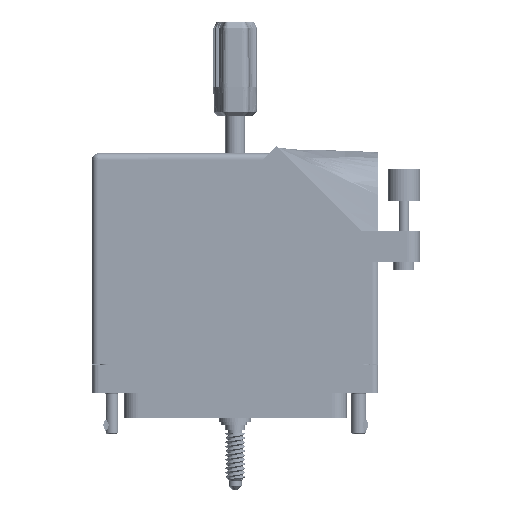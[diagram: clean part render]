
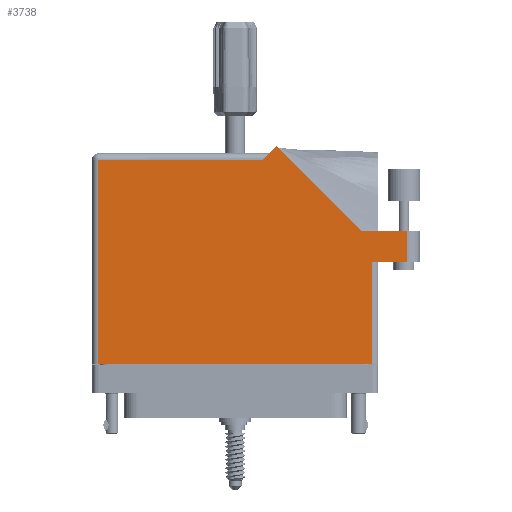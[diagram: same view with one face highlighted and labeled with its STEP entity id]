
A CAD part, front view. The second image highlights one B-rep face of the part: STEP entity #3738.
In plain terms, the highlighted face is planar.
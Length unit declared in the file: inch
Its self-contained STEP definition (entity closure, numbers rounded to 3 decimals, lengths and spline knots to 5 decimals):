
#2102 = ORIENTED_EDGE ( 'NONE', *, *, #64452, .T. ) ;
#3738 = ADVANCED_FACE ( 'NONE', ( #49669 ), #27587, .F. ) ;
#4021 = ORIENTED_EDGE ( 'NONE', *, *, #21366, .T. ) ;
#4444 = EDGE_CURVE ( 'NONE', #12340, #99884, #66323, .T. ) ;
#4753 = ORIENTED_EDGE ( 'NONE', *, *, #93222, .T. ) ;
#4767 = CARTESIAN_POINT ( 'NONE',  ( -1.3155, 1.868, 0.765 ) ) ;
#5941 = DIRECTION ( 'NONE',  ( -1., 0., 0. ) ) ;
#6833 = DIRECTION ( 'NONE',  ( -1., 0., 0. ) ) ;
#11622 = VECTOR ( 'NONE', #79929, 39.37008 ) ;
#11814 = VECTOR ( 'NONE', #38916, 39.37008 ) ;
#12340 = VERTEX_POINT ( 'NONE', #85760 ) ;
#12957 = VERTEX_POINT ( 'NONE', #61375 ) ;
#13577 = VERTEX_POINT ( 'NONE', #108773 ) ;
#13743 = CARTESIAN_POINT ( 'NONE',  ( 1.7775, 1.187, 0.765 ) ) ;
#15024 = CARTESIAN_POINT ( 'NONE',  ( -1.3775, 1.868, 0.765 ) ) ;
#18104 = DIRECTION ( 'NONE',  ( 0., -1., 0. ) ) ;
#18224 = LINE ( 'NONE', #71721, #22410 ) ;
#19710 = VERTEX_POINT ( 'NONE', #35113 ) ;
#21366 = EDGE_CURVE ( 'NONE', #12957, #83912, #101334, .T. ) ;
#21808 = VECTOR ( 'NONE', #59998, 39.37008 ) ;
#22410 = VECTOR ( 'NONE', #18104, 39.37008 ) ;
#23076 = CARTESIAN_POINT ( 'NONE',  ( 1.3775, 0.88, 0.765 ) ) ;
#27587 = PLANE ( 'NONE',  #37888 ) ;
#28535 = EDGE_LOOP ( 'NONE', ( #106718, #75778, #4021, #28876, #89731, #67244, #4753, #2102, #109315 ) ) ;
#28876 = ORIENTED_EDGE ( 'NONE', *, *, #99360, .T. ) ;
#32850 = LINE ( 'NONE', #23076, #11814 ) ;
#32872 = EDGE_CURVE ( 'NONE', #103027, #12340, #93542, .T. ) ;
#33157 = CARTESIAN_POINT ( 'NONE',  ( 0.3275, 1.93, 0.765 ) ) ;
#35113 = CARTESIAN_POINT ( 'NONE',  ( 1.6525, 0.88, 0.765 ) ) ;
#35695 = EDGE_CURVE ( 'NONE', #13577, #19710, #32850, .T. ) ;
#37389 = DIRECTION ( 'NONE',  ( 0., 0., -1. ) ) ;
#37735 = LINE ( 'NONE', #48229, #67104 ) ;
#37888 = AXIS2_PLACEMENT_3D ( 'NONE', #72532, #37389, #62780 ) ;
#38916 = DIRECTION ( 'NONE',  ( 1., 0., 0. ) ) ;
#43512 = LINE ( 'NONE', #103523, #61701 ) ;
#45171 = LINE ( 'NONE', #70104, #11622 ) ;
#46310 = VERTEX_POINT ( 'NONE', #104229 ) ;
#48229 = CARTESIAN_POINT ( 'NONE',  ( 1.6525, 1.187, 0.765 ) ) ;
#49669 = FACE_OUTER_BOUND ( 'NONE', #28535, .T. ) ;
#52642 = CARTESIAN_POINT ( 'NONE',  ( 1.21192, 1.187, 0.765 ) ) ;
#52667 = DIRECTION ( 'NONE',  ( -0.707, -0.707, 0. ) ) ;
#53614 = VECTOR ( 'NONE', #5941, 39.37008 ) ;
#59998 = DIRECTION ( 'NONE',  ( 0., 1., 0. ) ) ;
#61375 = CARTESIAN_POINT ( 'NONE',  ( 1.6525, 1.187, 0.765 ) ) ;
#61674 = EDGE_CURVE ( 'NONE', #46310, #13577, #72189, .T. ) ;
#61701 = VECTOR ( 'NONE', #66681, 39.37008 ) ;
#62780 = DIRECTION ( 'NONE',  ( -1., 0., 0. ) ) ;
#64452 = EDGE_CURVE ( 'NONE', #96827, #46310, #45171, .T. ) ;
#66323 = LINE ( 'NONE', #15024, #84586 ) ;
#66681 = DIRECTION ( 'NONE',  ( -0.707, 0.707, 0. ) ) ;
#67029 = EDGE_CURVE ( 'NONE', #19710, #12957, #37735, .T. ) ;
#67104 = VECTOR ( 'NONE', #112120, 39.37008 ) ;
#67244 = ORIENTED_EDGE ( 'NONE', *, *, #4444, .T. ) ;
#69595 = VECTOR ( 'NONE', #52667, 39.37008 ) ;
#70104 = CARTESIAN_POINT ( 'NONE',  ( -1.3775, -0.1, 0.765 ) ) ;
#71721 = CARTESIAN_POINT ( 'NONE',  ( -1.3155, -0.1, 0.765 ) ) ;
#72189 = LINE ( 'NONE', #114458, #21808 ) ;
#72532 = CARTESIAN_POINT ( 'NONE',  ( -1.3775, 1.93, 0.765 ) ) ;
#75778 = ORIENTED_EDGE ( 'NONE', *, *, #67029, .T. ) ;
#79929 = DIRECTION ( 'NONE',  ( 1., 0., 0. ) ) ;
#83912 = VERTEX_POINT ( 'NONE', #52642 ) ;
#84586 = VECTOR ( 'NONE', #6833, 39.37008 ) ;
#85760 = CARTESIAN_POINT ( 'NONE',  ( 0.2655, 1.868, 0.765 ) ) ;
#89337 = CARTESIAN_POINT ( 'NONE',  ( -1.3155, -0.1, 0.765 ) ) ;
#89731 = ORIENTED_EDGE ( 'NONE', *, *, #32872, .T. ) ;
#93222 = EDGE_CURVE ( 'NONE', #99884, #96827, #18224, .T. ) ;
#93542 = LINE ( 'NONE', #33157, #69595 ) ;
#96827 = VERTEX_POINT ( 'NONE', #89337 ) ;
#99360 = EDGE_CURVE ( 'NONE', #83912, #103027, #43512, .T. ) ;
#99884 = VERTEX_POINT ( 'NONE', #4767 ) ;
#101334 = LINE ( 'NONE', #13743, #53614 ) ;
#101834 = CARTESIAN_POINT ( 'NONE',  ( 0.39821, 2.00071, 0.765 ) ) ;
#103027 = VERTEX_POINT ( 'NONE', #101834 ) ;
#103523 = CARTESIAN_POINT ( 'NONE',  ( 1.21192, 1.187, 0.765 ) ) ;
#104229 = CARTESIAN_POINT ( 'NONE',  ( 1.3155, -0.1, 0.765 ) ) ;
#106718 = ORIENTED_EDGE ( 'NONE', *, *, #35695, .T. ) ;
#108773 = CARTESIAN_POINT ( 'NONE',  ( 1.3155, 0.88, 0.765 ) ) ;
#109315 = ORIENTED_EDGE ( 'NONE', *, *, #61674, .T. ) ;
#112120 = DIRECTION ( 'NONE',  ( 0., 1., 0. ) ) ;
#114458 = CARTESIAN_POINT ( 'NONE',  ( 1.3155, 0.88, 0.765 ) ) ;
